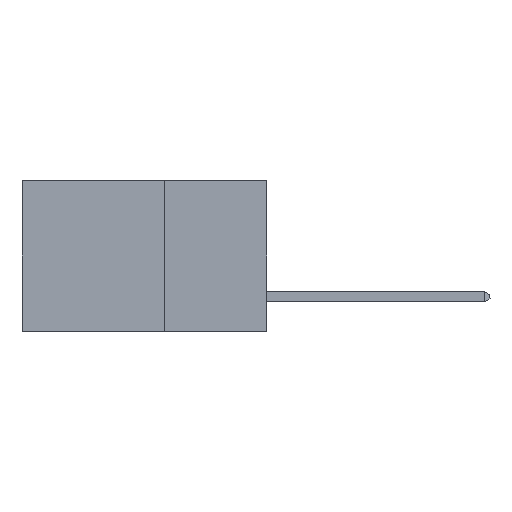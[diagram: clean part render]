
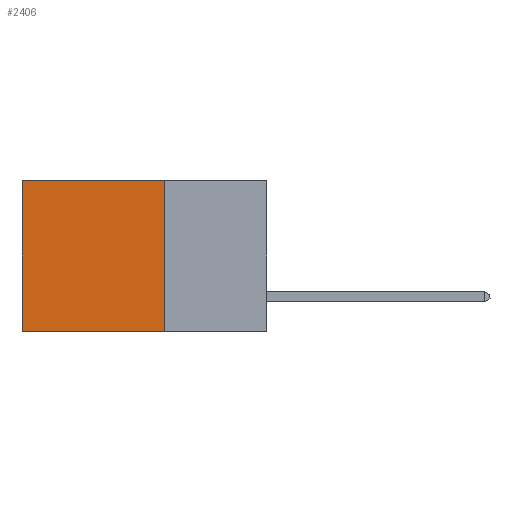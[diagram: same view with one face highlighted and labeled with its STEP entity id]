
A CAD part, left-side view. The second image highlights one B-rep face of the part: STEP entity #2406.
In plain terms, the highlighted planar face has unit normal (-1, 0, 0).
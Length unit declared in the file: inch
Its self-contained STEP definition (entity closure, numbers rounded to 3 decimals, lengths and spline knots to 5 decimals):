
#1143 = FACE_OUTER_BOUND ( 'NONE', #11468, .T. ) ;
#1477 = LINE ( 'NONE', #6835, #12155 ) ;
#1497 = VERTEX_POINT ( 'NONE', #3540 ) ;
#1518 = EDGE_CURVE ( 'NONE', #7773, #1497, #10568, .T. ) ;
#1540 = CARTESIAN_POINT ( 'NONE',  ( 0.2875, 0.25, -0.37 ) ) ;
#1745 = CARTESIAN_POINT ( 'NONE',  ( 0.2875, 0.25, 0. ) ) ;
#1779 = VERTEX_POINT ( 'NONE', #5089 ) ;
#2233 = CARTESIAN_POINT ( 'NONE',  ( 0.2875, 0.6, -0.37 ) ) ;
#2322 = VECTOR ( 'NONE', #11810, 39.37008 ) ;
#2325 = EDGE_CURVE ( 'NONE', #7773, #1779, #1477, .T. ) ;
#2406 = ADVANCED_FACE ( 'NONE', ( #1143 ), #7985, .F. ) ;
#2431 = VECTOR ( 'NONE', #3057, 39.37008 ) ;
#2798 = DIRECTION ( 'NONE',  ( 1., 0., 0. ) ) ;
#3057 = DIRECTION ( 'NONE',  ( 0., 0., -1. ) ) ;
#3540 = CARTESIAN_POINT ( 'NONE',  ( 0.2875, 0.25, -0.37 ) ) ;
#3577 = VECTOR ( 'NONE', #8869, 39.37008 ) ;
#3966 = VERTEX_POINT ( 'NONE', #2233 ) ;
#4481 = ORIENTED_EDGE ( 'NONE', *, *, #12874, .F. ) ;
#4980 = ORIENTED_EDGE ( 'NONE', *, *, #11036, .T. ) ;
#5089 = CARTESIAN_POINT ( 'NONE',  ( 0.2875, 0.6, 0. ) ) ;
#5234 = LINE ( 'NONE', #11300, #2431 ) ;
#5680 = ORIENTED_EDGE ( 'NONE', *, *, #1518, .F. ) ;
#6344 = LINE ( 'NONE', #1540, #3577 ) ;
#6551 = AXIS2_PLACEMENT_3D ( 'NONE', #1745, #2798, #10047 ) ;
#6835 = CARTESIAN_POINT ( 'NONE',  ( 0.2875, 0.25, 0. ) ) ;
#7753 = CARTESIAN_POINT ( 'NONE',  ( 0.2875, 0.25, 0. ) ) ;
#7773 = VERTEX_POINT ( 'NONE', #10885 ) ;
#7985 = PLANE ( 'NONE',  #6551 ) ;
#8869 = DIRECTION ( 'NONE',  ( 0., 1., 0. ) ) ;
#9981 = ORIENTED_EDGE ( 'NONE', *, *, #2325, .T. ) ;
#10047 = DIRECTION ( 'NONE',  ( 0., 0., -1. ) ) ;
#10568 = LINE ( 'NONE', #7753, #2322 ) ;
#10885 = CARTESIAN_POINT ( 'NONE',  ( 0.2875, 0.25, 0. ) ) ;
#11036 = EDGE_CURVE ( 'NONE', #1779, #3966, #5234, .T. ) ;
#11300 = CARTESIAN_POINT ( 'NONE',  ( 0.2875, 0.6, 0. ) ) ;
#11468 = EDGE_LOOP ( 'NONE', ( #4980, #4481, #5680, #9981 ) ) ;
#11810 = DIRECTION ( 'NONE',  ( 0., 0., -1. ) ) ;
#12155 = VECTOR ( 'NONE', #12957, 39.37008 ) ;
#12874 = EDGE_CURVE ( 'NONE', #1497, #3966, #6344, .T. ) ;
#12957 = DIRECTION ( 'NONE',  ( 0., 1., 0. ) ) ;
